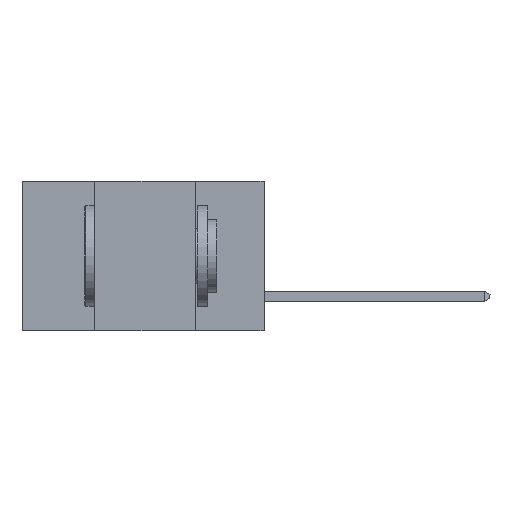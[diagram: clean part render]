
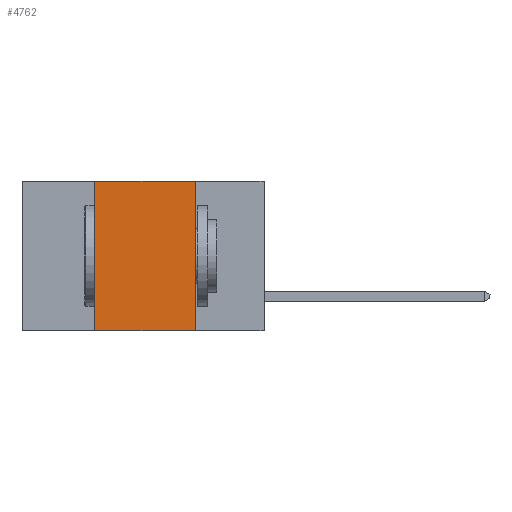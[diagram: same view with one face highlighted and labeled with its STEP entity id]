
A CAD part, left-side view. The second image highlights one B-rep face of the part: STEP entity #4762.
In plain terms, the highlighted planar face has unit normal (-1, 0, 0).
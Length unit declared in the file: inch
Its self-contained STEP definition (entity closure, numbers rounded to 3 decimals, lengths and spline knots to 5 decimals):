
#207 = CARTESIAN_POINT ( 'NONE',  ( 0., 0.6, 0. ) ) ;
#406 = LINE ( 'NONE', #4173, #4304 ) ;
#626 = CARTESIAN_POINT ( 'NONE',  ( 0., 0.17, 0. ) ) ;
#939 = DIRECTION ( 'NONE',  ( 0., -1., 0. ) ) ;
#1089 = CARTESIAN_POINT ( 'NONE',  ( 0., 0.17, -0.37 ) ) ;
#1910 = VERTEX_POINT ( 'NONE', #1089 ) ;
#1963 = CARTESIAN_POINT ( 'NONE',  ( 0., 0.42, 0. ) ) ;
#2086 = EDGE_CURVE ( 'NONE', #7192, #1910, #406, .T. ) ;
#3233 = FACE_OUTER_BOUND ( 'NONE', #6994, .T. ) ;
#3332 = DIRECTION ( 'NONE',  ( 1., 0., 0. ) ) ;
#3388 = DIRECTION ( 'NONE',  ( 0., -1., 0. ) ) ;
#3706 = ORIENTED_EDGE ( 'NONE', *, *, #4772, .F. ) ;
#3767 = ORIENTED_EDGE ( 'NONE', *, *, #7418, .F. ) ;
#4026 = CARTESIAN_POINT ( 'NONE',  ( 0., 0.17, -0.37 ) ) ;
#4173 = CARTESIAN_POINT ( 'NONE',  ( 0., 0.6, -0.37 ) ) ;
#4244 = LINE ( 'NONE', #9430, #8224 ) ;
#4304 = VECTOR ( 'NONE', #3388, 39.37008 ) ;
#4347 = VECTOR ( 'NONE', #4615, 39.37008 ) ;
#4615 = DIRECTION ( 'NONE',  ( 0., 0., -1. ) ) ;
#4741 = PLANE ( 'NONE',  #9441 ) ;
#4748 = LINE ( 'NONE', #4026, #4347 ) ;
#4762 = ADVANCED_FACE ( 'NONE', ( #3233 ), #4741, .F. ) ;
#4772 = EDGE_CURVE ( 'NONE', #6130, #5814, #6919, .T. ) ;
#5498 = ORIENTED_EDGE ( 'NONE', *, *, #6463, .F. ) ;
#5814 = VERTEX_POINT ( 'NONE', #626 ) ;
#6130 = VERTEX_POINT ( 'NONE', #1963 ) ;
#6149 = CARTESIAN_POINT ( 'NONE',  ( 0., 0.6, 0. ) ) ;
#6198 = DIRECTION ( 'NONE',  ( 0., 0., -1. ) ) ;
#6410 = DIRECTION ( 'NONE',  ( 0., 0., 1. ) ) ;
#6463 = EDGE_CURVE ( 'NONE', #5814, #1910, #4748, .T. ) ;
#6789 = VECTOR ( 'NONE', #939, 39.37008 ) ;
#6919 = LINE ( 'NONE', #6149, #6789 ) ;
#6994 = EDGE_LOOP ( 'NONE', ( #5498, #3706, #3767, #8069 ) ) ;
#7192 = VERTEX_POINT ( 'NONE', #7255 ) ;
#7255 = CARTESIAN_POINT ( 'NONE',  ( 0., 0.42, -0.37 ) ) ;
#7418 = EDGE_CURVE ( 'NONE', #7192, #6130, #4244, .T. ) ;
#8069 = ORIENTED_EDGE ( 'NONE', *, *, #2086, .T. ) ;
#8224 = VECTOR ( 'NONE', #6410, 39.37008 ) ;
#9430 = CARTESIAN_POINT ( 'NONE',  ( 0., 0.42, -0.37 ) ) ;
#9441 = AXIS2_PLACEMENT_3D ( 'NONE', #207, #3332, #6198 ) ;
